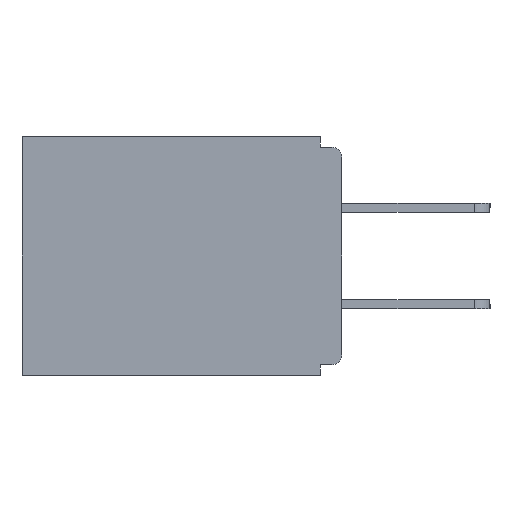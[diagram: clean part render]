
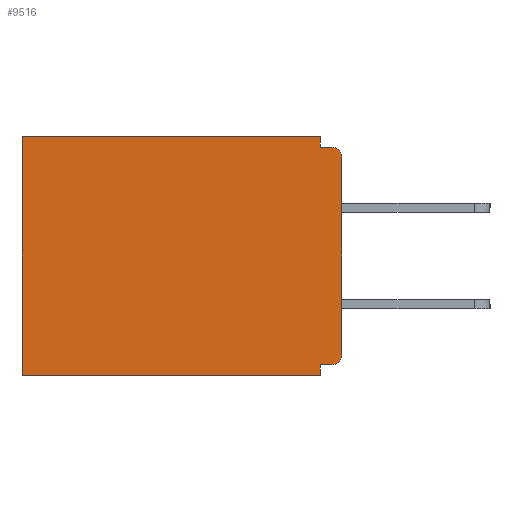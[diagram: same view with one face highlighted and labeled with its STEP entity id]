
A CAD part, left-side view. The second image highlights one B-rep face of the part: STEP entity #9516.
In plain terms, the highlighted planar face has unit normal (-1, 0, 0).
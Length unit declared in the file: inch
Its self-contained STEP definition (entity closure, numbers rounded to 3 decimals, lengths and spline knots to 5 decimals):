
#32 = VERTEX_POINT ( 'NONE', #397 ) ;
#264 = CIRCLE ( 'NONE', #2463, 0.015 ) ;
#286 = CARTESIAN_POINT ( 'NONE',  ( 0.298, 0.031, -0.015 ) ) ;
#393 = VERTEX_POINT ( 'NONE', #9179 ) ;
#397 = CARTESIAN_POINT ( 'NONE',  ( 0.298, 0.46, -0.343 ) ) ;
#425 = CARTESIAN_POINT ( 'NONE',  ( 0.298, 0.031, 0. ) ) ;
#627 = DIRECTION ( 'NONE',  ( 0., 0., -1. ) ) ;
#1008 = DIRECTION ( 'NONE',  ( 0., -1., 0. ) ) ;
#1173 = CIRCLE ( 'NONE', #13528, 0.015 ) ;
#1344 = CARTESIAN_POINT ( 'NONE',  ( 0.298, 0.015, -0.03 ) ) ;
#1347 = EDGE_CURVE ( 'NONE', #15143, #12449, #15703, .T. ) ;
#1359 = EDGE_CURVE ( 'NONE', #8782, #5039, #14021, .T. ) ;
#1500 = DIRECTION ( 'NONE',  ( 1., 0., 0. ) ) ;
#1575 = CARTESIAN_POINT ( 'NONE',  ( 0.298, 0., -0.328 ) ) ;
#1680 = LINE ( 'NONE', #11602, #5640 ) ;
#1698 = ORIENTED_EDGE ( 'NONE', *, *, #8710, .F. ) ;
#1710 = VECTOR ( 'NONE', #627, 39.37008 ) ;
#2379 = LINE ( 'NONE', #12556, #6745 ) ;
#2463 = AXIS2_PLACEMENT_3D ( 'NONE', #8664, #4688, #7316 ) ;
#2589 = CARTESIAN_POINT ( 'NONE',  ( 0.298, 0., 0. ) ) ;
#2665 = ORIENTED_EDGE ( 'NONE', *, *, #1359, .F. ) ;
#2922 = VECTOR ( 'NONE', #12435, 39.37008 ) ;
#3077 = VECTOR ( 'NONE', #12477, 39.37008 ) ;
#3262 = FACE_OUTER_BOUND ( 'NONE', #15092, .T. ) ;
#4517 = CARTESIAN_POINT ( 'NONE',  ( 0.298, 0.031, -0.343 ) ) ;
#4688 = DIRECTION ( 'NONE',  ( -1., 0., 0. ) ) ;
#5039 = VERTEX_POINT ( 'NONE', #7640 ) ;
#5442 = CARTESIAN_POINT ( 'NONE',  ( 0.298, 0., 0. ) ) ;
#5443 = CARTESIAN_POINT ( 'NONE',  ( 0.298, 0.031, -0.343 ) ) ;
#5508 = DIRECTION ( 'NONE',  ( 0., 0., -1. ) ) ;
#5640 = VECTOR ( 'NONE', #1008, 39.37008 ) ;
#5662 = AXIS2_PLACEMENT_3D ( 'NONE', #5442, #1500, #5508 ) ;
#5678 = CARTESIAN_POINT ( 'NONE',  ( 0.298, 0.015, -0.015 ) ) ;
#5691 = ORIENTED_EDGE ( 'NONE', *, *, #1347, .T. ) ;
#5811 = CARTESIAN_POINT ( 'NONE',  ( 0.298, 0., -0.343 ) ) ;
#5976 = EDGE_CURVE ( 'NONE', #8782, #7201, #1173, .T. ) ;
#6117 = EDGE_CURVE ( 'NONE', #11176, #7446, #14072, .T. ) ;
#6450 = LINE ( 'NONE', #5811, #2922 ) ;
#6467 = ORIENTED_EDGE ( 'NONE', *, *, #13883, .F. ) ;
#6507 = DIRECTION ( 'NONE',  ( 0., 0., -1. ) ) ;
#6745 = VECTOR ( 'NONE', #16388, 39.37008 ) ;
#7201 = VERTEX_POINT ( 'NONE', #5678 ) ;
#7316 = DIRECTION ( 'NONE',  ( 0., 0., -1. ) ) ;
#7446 = VERTEX_POINT ( 'NONE', #13039 ) ;
#7572 = EDGE_CURVE ( 'NONE', #9289, #7201, #1680, .T. ) ;
#7640 = CARTESIAN_POINT ( 'NONE',  ( 0.298, 0., -0.313 ) ) ;
#7696 = CARTESIAN_POINT ( 'NONE',  ( 0.298, 0.015, -0.328 ) ) ;
#8196 = VECTOR ( 'NONE', #11895, 39.37008 ) ;
#8664 = CARTESIAN_POINT ( 'NONE',  ( 0.298, 0.015, -0.313 ) ) ;
#8710 = EDGE_CURVE ( 'NONE', #15143, #9289, #13487, .T. ) ;
#8782 = VERTEX_POINT ( 'NONE', #9687 ) ;
#8848 = ORIENTED_EDGE ( 'NONE', *, *, #14755, .F. ) ;
#9179 = CARTESIAN_POINT ( 'NONE',  ( 0.298, 0.031, -0.343 ) ) ;
#9289 = VERTEX_POINT ( 'NONE', #286 ) ;
#9312 = ORIENTED_EDGE ( 'NONE', *, *, #5976, .T. ) ;
#9516 = ADVANCED_FACE ( 'NONE', ( #3262 ), #14581, .F. ) ;
#9687 = CARTESIAN_POINT ( 'NONE',  ( 0.298, 0., -0.03 ) ) ;
#10420 = ORIENTED_EDGE ( 'NONE', *, *, #13838, .T. ) ;
#10540 = DIRECTION ( 'NONE',  ( 0., 1., 0. ) ) ;
#10564 = DIRECTION ( 'NONE',  ( -1., 0., 0. ) ) ;
#10738 = EDGE_CURVE ( 'NONE', #12449, #32, #2379, .T. ) ;
#11176 = VERTEX_POINT ( 'NONE', #7696 ) ;
#11380 = VECTOR ( 'NONE', #12147, 39.37008 ) ;
#11602 = CARTESIAN_POINT ( 'NONE',  ( 0.298, 0., -0.015 ) ) ;
#11895 = DIRECTION ( 'NONE',  ( 0., 0., -1. ) ) ;
#12147 = DIRECTION ( 'NONE',  ( 0., 1., 0. ) ) ;
#12341 = VECTOR ( 'NONE', #10540, 39.37008 ) ;
#12435 = DIRECTION ( 'NONE',  ( 0., 1., 0. ) ) ;
#12449 = VERTEX_POINT ( 'NONE', #13873 ) ;
#12477 = DIRECTION ( 'NONE',  ( 0., 0., -1. ) ) ;
#12556 = CARTESIAN_POINT ( 'NONE',  ( 0.298, 0.46, 0. ) ) ;
#13039 = CARTESIAN_POINT ( 'NONE',  ( 0.298, 0.031, -0.328 ) ) ;
#13487 = LINE ( 'NONE', #5443, #3077 ) ;
#13528 = AXIS2_PLACEMENT_3D ( 'NONE', #1344, #10564, #6507 ) ;
#13838 = EDGE_CURVE ( 'NONE', #11176, #5039, #264, .T. ) ;
#13873 = CARTESIAN_POINT ( 'NONE',  ( 0.298, 0.46, 0. ) ) ;
#13883 = EDGE_CURVE ( 'NONE', #7446, #393, #15865, .T. ) ;
#14021 = LINE ( 'NONE', #17184, #8196 ) ;
#14072 = LINE ( 'NONE', #1575, #11380 ) ;
#14081 = ORIENTED_EDGE ( 'NONE', *, *, #10738, .T. ) ;
#14089 = ORIENTED_EDGE ( 'NONE', *, *, #6117, .F. ) ;
#14581 = PLANE ( 'NONE',  #5662 ) ;
#14755 = EDGE_CURVE ( 'NONE', #393, #32, #6450, .T. ) ;
#14965 = ORIENTED_EDGE ( 'NONE', *, *, #7572, .F. ) ;
#15092 = EDGE_LOOP ( 'NONE', ( #9312, #14965, #1698, #5691, #14081, #8848, #6467, #14089, #10420, #2665 ) ) ;
#15143 = VERTEX_POINT ( 'NONE', #425 ) ;
#15703 = LINE ( 'NONE', #2589, #12341 ) ;
#15865 = LINE ( 'NONE', #4517, #1710 ) ;
#16388 = DIRECTION ( 'NONE',  ( 0., 0., -1. ) ) ;
#17184 = CARTESIAN_POINT ( 'NONE',  ( 0.298, 0., 0. ) ) ;
